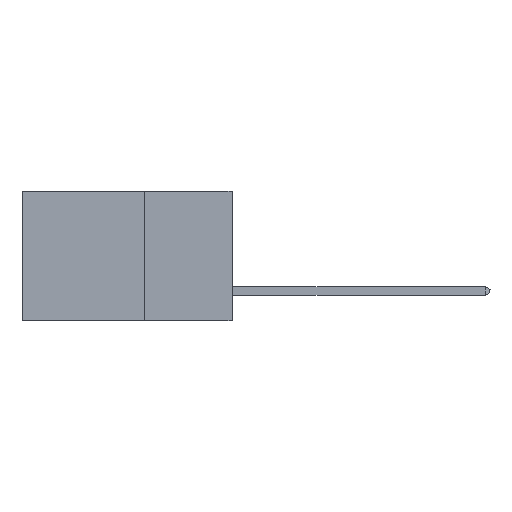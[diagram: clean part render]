
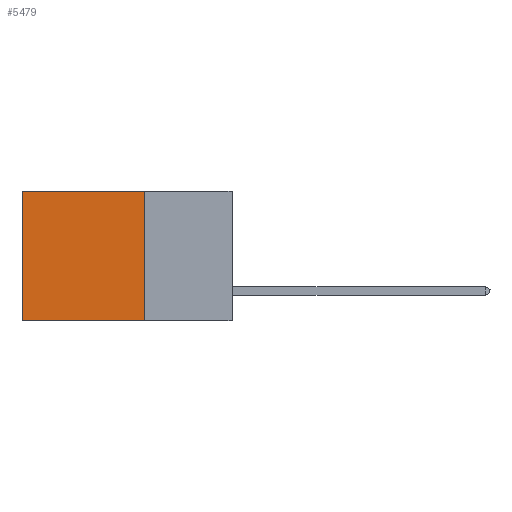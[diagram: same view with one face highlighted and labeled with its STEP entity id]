
A CAD part, left-side view. The second image highlights one B-rep face of the part: STEP entity #5479.
In plain terms, the highlighted planar face has unit normal (-1, 0, 0).
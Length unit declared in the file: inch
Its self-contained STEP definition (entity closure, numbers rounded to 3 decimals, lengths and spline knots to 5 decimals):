
#1058 = LINE ( 'NONE', #29948, #12886 ) ;
#1109 = FACE_OUTER_BOUND ( 'NONE', #28318, .T. ) ;
#2179 = VERTEX_POINT ( 'NONE', #15828 ) ;
#3307 = ORIENTED_EDGE ( 'NONE', *, *, #27094, .T. ) ;
#3848 = CARTESIAN_POINT ( 'NONE',  ( 0.2875, 0.25, 0. ) ) ;
#4210 = DIRECTION ( 'NONE',  ( 0., 0., -1. ) ) ;
#5479 = ADVANCED_FACE ( 'NONE', ( #1109 ), #22952, .F. ) ;
#7251 = EDGE_CURVE ( 'NONE', #21242, #2179, #37510, .T. ) ;
#7706 = ORIENTED_EDGE ( 'NONE', *, *, #7251, .F. ) ;
#8536 = DIRECTION ( 'NONE',  ( 0., 0., -1. ) ) ;
#9813 = VECTOR ( 'NONE', #24511, 39.37008 ) ;
#12886 = VECTOR ( 'NONE', #15642, 39.37008 ) ;
#13597 = ORIENTED_EDGE ( 'NONE', *, *, #28809, .F. ) ;
#13870 = DIRECTION ( 'NONE',  ( 0., 1., 0. ) ) ;
#14646 = VECTOR ( 'NONE', #4210, 39.37008 ) ;
#15642 = DIRECTION ( 'NONE',  ( 0., 0., -1. ) ) ;
#15828 = CARTESIAN_POINT ( 'NONE',  ( 0.2875, 0.25, -0.37 ) ) ;
#17224 = DIRECTION ( 'NONE',  ( 1., 0., 0. ) ) ;
#17567 = CARTESIAN_POINT ( 'NONE',  ( 0.2875, 0.6, 0. ) ) ;
#18787 = VECTOR ( 'NONE', #13870, 39.37008 ) ;
#18882 = VERTEX_POINT ( 'NONE', #19151 ) ;
#19151 = CARTESIAN_POINT ( 'NONE',  ( 0.2875, 0.6, -0.37 ) ) ;
#19798 = VERTEX_POINT ( 'NONE', #17567 ) ;
#20394 = CARTESIAN_POINT ( 'NONE',  ( 0.2875, 0.25, 0. ) ) ;
#21242 = VERTEX_POINT ( 'NONE', #3848 ) ;
#22952 = PLANE ( 'NONE',  #31874 ) ;
#24511 = DIRECTION ( 'NONE',  ( 0., 1., 0. ) ) ;
#26302 = LINE ( 'NONE', #33559, #9813 ) ;
#27094 = EDGE_CURVE ( 'NONE', #19798, #18882, #1058, .T. ) ;
#27927 = LINE ( 'NONE', #31373, #18787 ) ;
#28318 = EDGE_LOOP ( 'NONE', ( #3307, #13597, #7706, #28349 ) ) ;
#28349 = ORIENTED_EDGE ( 'NONE', *, *, #32362, .T. ) ;
#28809 = EDGE_CURVE ( 'NONE', #2179, #18882, #27927, .T. ) ;
#29948 = CARTESIAN_POINT ( 'NONE',  ( 0.2875, 0.6, 0. ) ) ;
#30817 = CARTESIAN_POINT ( 'NONE',  ( 0.2875, 0.25, 0. ) ) ;
#31373 = CARTESIAN_POINT ( 'NONE',  ( 0.2875, 0.25, -0.37 ) ) ;
#31874 = AXIS2_PLACEMENT_3D ( 'NONE', #20394, #17224, #8536 ) ;
#32362 = EDGE_CURVE ( 'NONE', #21242, #19798, #26302, .T. ) ;
#33559 = CARTESIAN_POINT ( 'NONE',  ( 0.2875, 0.25, 0. ) ) ;
#37510 = LINE ( 'NONE', #30817, #14646 ) ;
